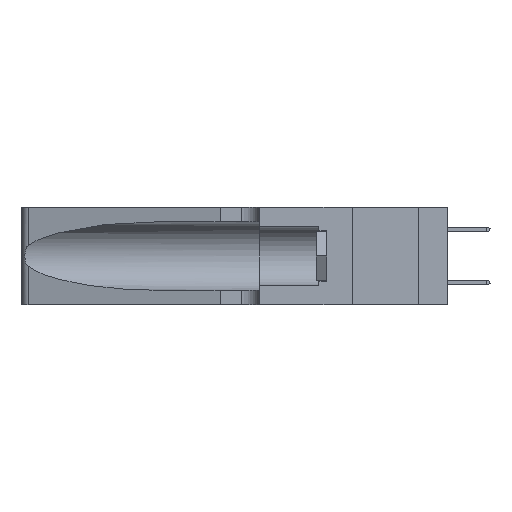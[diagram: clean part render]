
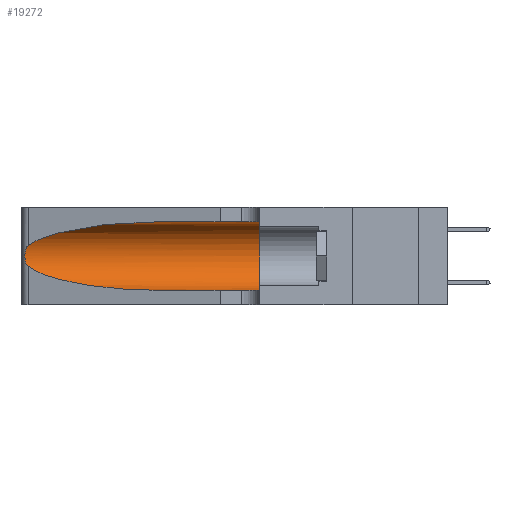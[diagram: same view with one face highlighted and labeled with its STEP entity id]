
A CAD part, left-side view. The second image highlights one B-rep face of the part: STEP entity #19272.
In plain terms, the highlighted cylindrical face has radius 3.308 mm (diameter 6.617 mm), a partial arc.
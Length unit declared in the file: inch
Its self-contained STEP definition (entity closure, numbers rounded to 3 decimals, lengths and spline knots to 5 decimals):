
#208 = ORIENTED_EDGE ( 'NONE', *, *, #2366, .T. ) ;
#842 = ORIENTED_EDGE ( 'NONE', *, *, #8107, .T. ) ;
#843 = DIRECTION ( 'NONE',  ( 0., 1., 0. ) ) ;
#1057 = CARTESIAN_POINT ( 'NONE',  ( 0.25856, 1.23593, 0.16098 ) ) ;
#1374 = CARTESIAN_POINT ( 'NONE',  ( 0.2373, 1.15595, 0.28018 ) ) ;
#1437 = CARTESIAN_POINT ( 'NONE',  ( 0.1305, 0.35, 0.31525 ) ) ;
#1565 = CARTESIAN_POINT ( 'NONE',  ( 0.25487, 1.22718, 0.14631 ) ) ;
#1872 = VERTEX_POINT ( 'NONE', #1882 ) ;
#1882 = CARTESIAN_POINT ( 'NONE',  ( 0.25487, 1.22718, 0.14631 ) ) ;
#2366 = EDGE_CURVE ( 'NONE', #9372, #5053, #5395, .T. ) ;
#2662 = CARTESIAN_POINT ( 'NONE',  ( 0.25639, 1.23186, 0.15144 ) ) ;
#2725 = CARTESIAN_POINT ( 'NONE',  ( 0.1305, 0.35, 0.05475 ) ) ;
#2862 = AXIS2_PLACEMENT_3D ( 'NONE', #10007, #843, #11549 ) ;
#3042 = LINE ( 'NONE', #11247, #18639 ) ;
#3084 = CARTESIAN_POINT ( 'NONE',  ( 0.1305, 1.61858, 0.05475 ) ) ;
#3162 = CARTESIAN_POINT ( 'NONE',  ( 0.18966, 0.96281, 0.05475 ) ) ;
#3462 = LINE ( 'NONE', #3084, #15045 ) ;
#3495 = ORIENTED_EDGE ( 'NONE', *, *, #4085, .F. ) ;
#4085 = EDGE_CURVE ( 'NONE', #15316, #19719, #11397, .T. ) ;
#4172 = CARTESIAN_POINT ( 'NONE',  ( 0.25555, 1.22994, 0.2215 ) ) ;
#4238 = CARTESIAN_POINT ( 'NONE',  ( 0.25487, 1.22718, 0.14631 ) ) ;
#4584 = EDGE_CURVE ( 'NONE', #5053, #1872, #19703, .T. ) ;
#5053 = VERTEX_POINT ( 'NONE', #17299 ) ;
#5395 =( BOUNDED_CURVE ( )  B_SPLINE_CURVE ( 3, ( #10525, #19541, #1374, #12067 ),
 .UNSPECIFIED., .F., .T. ) 
 B_SPLINE_CURVE_WITH_KNOTS ( ( 4, 4 ),
 ( 1.5708, 2.84003 ),
 .UNSPECIFIED. ) 
 CURVE ( )  GEOMETRIC_REPRESENTATION_ITEM ( )  RATIONAL_B_SPLINE_CURVE ( ( 1., 0.87, 0.87, 1. ) ) 
 REPRESENTATION_ITEM ( '' )  );
#5628 = EDGE_CURVE ( 'NONE', #9372, #15316, #3042, .T. ) ;
#5682 = CARTESIAN_POINT ( 'NONE',  ( 0.25639, 1.23184, 0.21858 ) ) ;
#7193 = CARTESIAN_POINT ( 'NONE',  ( 0.25854, 1.2359, 0.20912 ) ) ;
#7998 = CARTESIAN_POINT ( 'NONE',  ( 0.1305, 0.72297, 0.05475 ) ) ;
#8107 = EDGE_CURVE ( 'NONE', #16752, #19719, #3462, .T. ) ;
#8633 = CARTESIAN_POINT ( 'NONE',  ( 0.25487, 1.22718, 0.22369 ) ) ;
#8699 = CARTESIAN_POINT ( 'NONE',  ( 0.26075, 1.23896, 0.19203 ) ) ;
#9236 = ORIENTED_EDGE ( 'NONE', *, *, #17281, .T. ) ;
#9366 =( BOUNDED_CURVE ( )  B_SPLINE_CURVE ( 3, ( #1565, #10695, #3162, #13752 ),
 .UNSPECIFIED., .F., .F. ) 
 B_SPLINE_CURVE_WITH_KNOTS ( ( 4, 4 ),
 ( 3.44316, 4.71239 ),
 .UNSPECIFIED. ) 
 CURVE ( )  GEOMETRIC_REPRESENTATION_ITEM ( )  RATIONAL_B_SPLINE_CURVE ( ( 1., 0.87, 0.87, 1. ) ) 
 REPRESENTATION_ITEM ( '' )  );
#9372 = VERTEX_POINT ( 'NONE', #13890 ) ;
#9710 = DIRECTION ( 'NONE',  ( 0., -1., 0. ) ) ;
#10007 = CARTESIAN_POINT ( 'NONE',  ( 0.1305, 0.35, 0.185 ) ) ;
#10217 = CARTESIAN_POINT ( 'NONE',  ( 0.26017, 1.23833, 0.17102 ) ) ;
#10525 = CARTESIAN_POINT ( 'NONE',  ( 0.1305, 0.72297, 0.31525 ) ) ;
#10621 = DIRECTION ( 'NONE',  ( 0., -1., 0. ) ) ;
#10695 = CARTESIAN_POINT ( 'NONE',  ( 0.2373, 1.15595, 0.08982 ) ) ;
#11247 = CARTESIAN_POINT ( 'NONE',  ( 0.1305, 1.61858, 0.31525 ) ) ;
#11397 = CIRCLE ( 'NONE', #2862, 0.13025 ) ;
#11549 = DIRECTION ( 'NONE',  ( 0., 0., 1. ) ) ;
#11753 = CARTESIAN_POINT ( 'NONE',  ( 0.25789, 1.23486, 0.15765 ) ) ;
#12067 = CARTESIAN_POINT ( 'NONE',  ( 0.25487, 1.22718, 0.22369 ) ) ;
#12125 = FACE_OUTER_BOUND ( 'NONE', #14837, .T. ) ;
#13277 = CARTESIAN_POINT ( 'NONE',  ( 0.25555, 1.22993, 0.14849 ) ) ;
#13480 = ORIENTED_EDGE ( 'NONE', *, *, #4584, .T. ) ;
#13752 = CARTESIAN_POINT ( 'NONE',  ( 0.1305, 0.72297, 0.05475 ) ) ;
#13869 = DIRECTION ( 'NONE',  ( 0., -1., 0. ) ) ;
#13890 = CARTESIAN_POINT ( 'NONE',  ( 0.1305, 0.72297, 0.31525 ) ) ;
#14837 = EDGE_LOOP ( 'NONE', ( #208, #13480, #9236, #842, #3495, #16210 ) ) ;
#15045 = VECTOR ( 'NONE', #10621, 39.37008 ) ;
#15316 = VERTEX_POINT ( 'NONE', #1437 ) ;
#15393 = CARTESIAN_POINT ( 'NONE',  ( 0.1305, 1.61858, 0.185 ) ) ;
#15660 = CYLINDRICAL_SURFACE ( 'NONE', #15752, 0.13025 ) ;
#15752 = AXIS2_PLACEMENT_3D ( 'NONE', #15393, #13869, #16918 ) ;
#16210 = ORIENTED_EDGE ( 'NONE', *, *, #5628, .F. ) ;
#16258 = CARTESIAN_POINT ( 'NONE',  ( 0.25787, 1.23484, 0.2124 ) ) ;
#16752 = VERTEX_POINT ( 'NONE', #7998 ) ;
#16918 = DIRECTION ( 'NONE',  ( 0., 0., -1. ) ) ;
#17281 = EDGE_CURVE ( 'NONE', #1872, #16752, #9366, .T. ) ;
#17299 = CARTESIAN_POINT ( 'NONE',  ( 0.25487, 1.22718, 0.22369 ) ) ;
#17769 = CARTESIAN_POINT ( 'NONE',  ( 0.26018, 1.23835, 0.19895 ) ) ;
#18639 = VECTOR ( 'NONE', #9710, 39.37008 ) ;
#19259 = CARTESIAN_POINT ( 'NONE',  ( 0.26075, 1.23896, 0.178 ) ) ;
#19272 = ADVANCED_FACE ( 'NONE', ( #12125 ), #15660, .F. ) ;
#19541 = CARTESIAN_POINT ( 'NONE',  ( 0.18966, 0.96281, 0.31525 ) ) ;
#19703 = B_SPLINE_CURVE_WITH_KNOTS ( 'NONE', 3,
 ( #8633, #4172, #5682, #16258, #7193, #17769, #8699, #19259, #10217, #1057, #11753, #2662, #13277, #4238 ),
 .UNSPECIFIED., .F., .F.,
 ( 4, 2, 2, 2, 2, 2, 4 ),
 ( 0., 0.00027, 0.00053, 0.00107, 0.0016, 0.00187, 0.00214 ),
 .UNSPECIFIED. ) ;
#19719 = VERTEX_POINT ( 'NONE', #2725 ) ;
